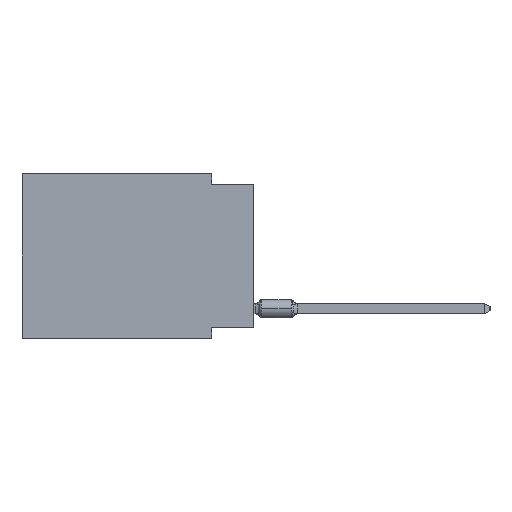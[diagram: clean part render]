
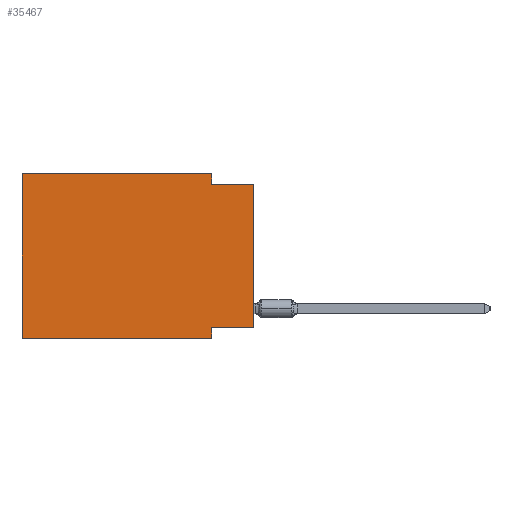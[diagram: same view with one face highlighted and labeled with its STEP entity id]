
A CAD part, left-side view. The second image highlights one B-rep face of the part: STEP entity #35467.
In plain terms, the highlighted planar face has unit normal (-1, 0, 0).
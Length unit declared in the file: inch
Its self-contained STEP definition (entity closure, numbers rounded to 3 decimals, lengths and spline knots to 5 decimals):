
#914 = FACE_OUTER_BOUND ( 'NONE', #23498, .T. ) ;
#1057 = DIRECTION ( 'NONE',  ( 0., 0., -1. ) ) ;
#1352 = LINE ( 'NONE', #58219, #2220 ) ;
#2220 = VECTOR ( 'NONE', #1057, 39.37008 ) ;
#2616 = CARTESIAN_POINT ( 'NONE',  ( 0., 0.55, 0. ) ) ;
#3581 = VERTEX_POINT ( 'NONE', #18869 ) ;
#3589 = LINE ( 'NONE', #37497, #59392 ) ;
#5568 = DIRECTION ( 'NONE',  ( 0., 0., -1. ) ) ;
#6561 = VERTEX_POINT ( 'NONE', #13025 ) ;
#9201 = EDGE_CURVE ( 'NONE', #60341, #41867, #43279, .T. ) ;
#9347 = CARTESIAN_POINT ( 'NONE',  ( 0., 0.1, 0. ) ) ;
#11439 = VECTOR ( 'NONE', #12889, 39.37008 ) ;
#11706 = LINE ( 'NONE', #2616, #13791 ) ;
#12889 = DIRECTION ( 'NONE',  ( 0., -1., 0. ) ) ;
#13025 = CARTESIAN_POINT ( 'NONE',  ( 0., 0., -0.365 ) ) ;
#13135 = EDGE_CURVE ( 'NONE', #41867, #45969, #46815, .T. ) ;
#13791 = VECTOR ( 'NONE', #21757, 39.37008 ) ;
#14718 = DIRECTION ( 'NONE',  ( 0., 1., 0. ) ) ;
#15857 = EDGE_CURVE ( 'NONE', #6561, #24200, #30111, .T. ) ;
#16420 = VECTOR ( 'NONE', #16471, 39.37008 ) ;
#16471 = DIRECTION ( 'NONE',  ( 0., 0., 1. ) ) ;
#16889 = EDGE_CURVE ( 'NONE', #58195, #25437, #11706, .T. ) ;
#18869 = CARTESIAN_POINT ( 'NONE',  ( 0., 0.1, -0.39 ) ) ;
#19862 = VECTOR ( 'NONE', #14718, 39.37008 ) ;
#20365 = CARTESIAN_POINT ( 'NONE',  ( 0., 0., -0.365 ) ) ;
#20706 = ORIENTED_EDGE ( 'NONE', *, *, #23664, .F. ) ;
#21757 = DIRECTION ( 'NONE',  ( 0., 0., 1. ) ) ;
#22558 = ORIENTED_EDGE ( 'NONE', *, *, #27610, .T. ) ;
#22816 = ORIENTED_EDGE ( 'NONE', *, *, #9201, .F. ) ;
#23498 = EDGE_LOOP ( 'NONE', ( #22558, #29706, #22816, #20706, #52678, #27234, #48916, #33105 ) ) ;
#23664 = EDGE_CURVE ( 'NONE', #25437, #60341, #3589, .T. ) ;
#24200 = VERTEX_POINT ( 'NONE', #31176 ) ;
#25437 = VERTEX_POINT ( 'NONE', #33979 ) ;
#26927 = EDGE_CURVE ( 'NONE', #58195, #3581, #31775, .T. ) ;
#27234 = ORIENTED_EDGE ( 'NONE', *, *, #26927, .T. ) ;
#27610 = EDGE_CURVE ( 'NONE', #6561, #45969, #39437, .T. ) ;
#28682 = AXIS2_PLACEMENT_3D ( 'NONE', #33260, #33578, #29482 ) ;
#29482 = DIRECTION ( 'NONE',  ( 0., 0., -1. ) ) ;
#29706 = ORIENTED_EDGE ( 'NONE', *, *, #13135, .F. ) ;
#30111 = LINE ( 'NONE', #20365, #19862 ) ;
#31176 = CARTESIAN_POINT ( 'NONE',  ( 0., 0.1, -0.365 ) ) ;
#31206 = EDGE_CURVE ( 'NONE', #24200, #3581, #1352, .T. ) ;
#31775 = LINE ( 'NONE', #45606, #43489 ) ;
#33105 = ORIENTED_EDGE ( 'NONE', *, *, #15857, .F. ) ;
#33260 = CARTESIAN_POINT ( 'NONE',  ( 0., 0.55, 0. ) ) ;
#33578 = DIRECTION ( 'NONE',  ( 1., 0., 0. ) ) ;
#33979 = CARTESIAN_POINT ( 'NONE',  ( 0., 0.55, 0. ) ) ;
#35467 = ADVANCED_FACE ( 'NONE', ( #914 ), #47722, .F. ) ;
#36770 = CARTESIAN_POINT ( 'NONE',  ( 0., 0., -0.025 ) ) ;
#37497 = CARTESIAN_POINT ( 'NONE',  ( 0., 0.55, 0. ) ) ;
#39437 = LINE ( 'NONE', #58895, #16420 ) ;
#41183 = CARTESIAN_POINT ( 'NONE',  ( 0., 0.1, -0.025 ) ) ;
#41867 = VERTEX_POINT ( 'NONE', #41183 ) ;
#43279 = LINE ( 'NONE', #9347, #57298 ) ;
#43489 = VECTOR ( 'NONE', #54730, 39.37008 ) ;
#45606 = CARTESIAN_POINT ( 'NONE',  ( 0., 0.55, -0.39 ) ) ;
#45637 = CARTESIAN_POINT ( 'NONE',  ( 0., 0., -0.025 ) ) ;
#45969 = VERTEX_POINT ( 'NONE', #45637 ) ;
#46319 = DIRECTION ( 'NONE',  ( 0., -1., 0. ) ) ;
#46815 = LINE ( 'NONE', #36770, #11439 ) ;
#47722 = PLANE ( 'NONE',  #28682 ) ;
#47976 = CARTESIAN_POINT ( 'NONE',  ( 0., 0.1, 0. ) ) ;
#48916 = ORIENTED_EDGE ( 'NONE', *, *, #31206, .F. ) ;
#52678 = ORIENTED_EDGE ( 'NONE', *, *, #16889, .F. ) ;
#54730 = DIRECTION ( 'NONE',  ( 0., -1., 0. ) ) ;
#57298 = VECTOR ( 'NONE', #5568, 39.37008 ) ;
#58195 = VERTEX_POINT ( 'NONE', #58859 ) ;
#58219 = CARTESIAN_POINT ( 'NONE',  ( 0., 0.1, -0.39 ) ) ;
#58859 = CARTESIAN_POINT ( 'NONE',  ( 0., 0.55, -0.39 ) ) ;
#58895 = CARTESIAN_POINT ( 'NONE',  ( 0., 0., 0. ) ) ;
#59392 = VECTOR ( 'NONE', #46319, 39.37008 ) ;
#60341 = VERTEX_POINT ( 'NONE', #47976 ) ;
